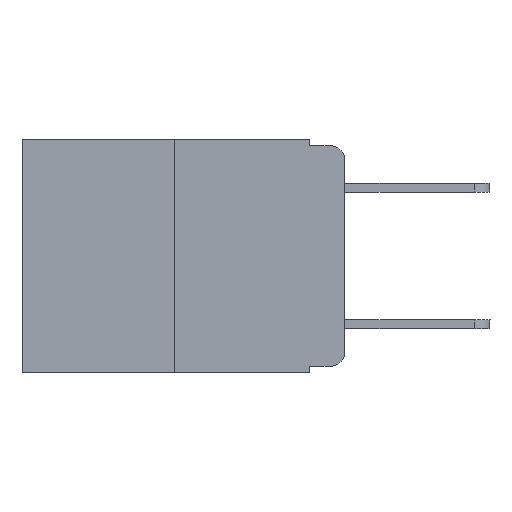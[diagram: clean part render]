
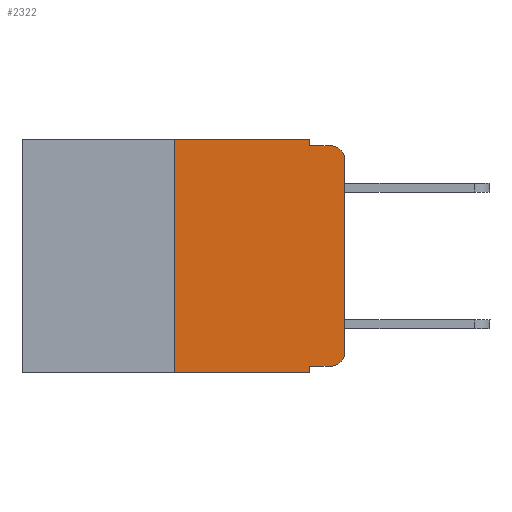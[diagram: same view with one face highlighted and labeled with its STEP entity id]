
A CAD part, left-side view. The second image highlights one B-rep face of the part: STEP entity #2322.
In plain terms, the highlighted planar face has unit normal (-1, 0, 0).
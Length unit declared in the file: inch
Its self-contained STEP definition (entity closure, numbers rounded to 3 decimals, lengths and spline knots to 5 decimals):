
#165 = VERTEX_POINT ( 'NONE', #23968 ) ;
#186 = VERTEX_POINT ( 'NONE', #12737 ) ;
#505 = VECTOR ( 'NONE', #11627, 39.37008 ) ;
#520 = EDGE_CURVE ( 'NONE', #7403, #3630, #7107, .T. ) ;
#828 = DIRECTION ( 'NONE',  ( -1., 0., 0. ) ) ;
#853 = ORIENTED_EDGE ( 'NONE', *, *, #20321, .T. ) ;
#989 = CARTESIAN_POINT ( 'NONE',  ( 0., 0.051, 0. ) ) ;
#1106 = EDGE_CURVE ( 'NONE', #11056, #7403, #2217, .T. ) ;
#1409 = EDGE_CURVE ( 'NONE', #17975, #5112, #13227, .T. ) ;
#1468 = VECTOR ( 'NONE', #15416, 39.37008 ) ;
#1956 = CARTESIAN_POINT ( 'NONE',  ( 0., 0.02, -0.03 ) ) ;
#1979 = VECTOR ( 'NONE', #15609, 39.37008 ) ;
#2217 = LINE ( 'NONE', #9827, #9112 ) ;
#2223 = VECTOR ( 'NONE', #4054, 39.37008 ) ;
#2322 = ADVANCED_FACE ( 'NONE', ( #21819 ), #15921, .F. ) ;
#2340 = CARTESIAN_POINT ( 'NONE',  ( 0., 0.25, -0.343 ) ) ;
#2586 = CARTESIAN_POINT ( 'NONE',  ( 0., 0.051, -0.01 ) ) ;
#2604 = VECTOR ( 'NONE', #2960, 39.37008 ) ;
#2744 = ORIENTED_EDGE ( 'NONE', *, *, #22276, .T. ) ;
#2960 = DIRECTION ( 'NONE',  ( 0., -1., 0. ) ) ;
#3630 = VERTEX_POINT ( 'NONE', #23465 ) ;
#4054 = DIRECTION ( 'NONE',  ( 0., 0., 1. ) ) ;
#4365 = CARTESIAN_POINT ( 'NONE',  ( 0., 0.051, 0. ) ) ;
#4501 = EDGE_CURVE ( 'NONE', #16630, #186, #10085, .T. ) ;
#5112 = VERTEX_POINT ( 'NONE', #14822 ) ;
#5150 = ORIENTED_EDGE ( 'NONE', *, *, #1106, .T. ) ;
#5334 = CARTESIAN_POINT ( 'NONE',  ( 0., 0.051, -0.333 ) ) ;
#5930 = AXIS2_PLACEMENT_3D ( 'NONE', #19654, #17916, #14220 ) ;
#6317 = ORIENTED_EDGE ( 'NONE', *, *, #18060, .F. ) ;
#6747 = ORIENTED_EDGE ( 'NONE', *, *, #4501, .F. ) ;
#6922 = ORIENTED_EDGE ( 'NONE', *, *, #520, .T. ) ;
#7107 = CIRCLE ( 'NONE', #5930, 0.02 ) ;
#7403 = VERTEX_POINT ( 'NONE', #7858 ) ;
#7858 = CARTESIAN_POINT ( 'NONE',  ( 0., 0.02, -0.333 ) ) ;
#8800 = DIRECTION ( 'NONE',  ( 0., 0., 1. ) ) ;
#9112 = VECTOR ( 'NONE', #18946, 39.37008 ) ;
#9827 = CARTESIAN_POINT ( 'NONE',  ( 0., 0.051, -0.333 ) ) ;
#10085 = LINE ( 'NONE', #989, #14245 ) ;
#10498 = DIRECTION ( 'NONE',  ( 0., 0., -1. ) ) ;
#11056 = VERTEX_POINT ( 'NONE', #5334 ) ;
#11627 = DIRECTION ( 'NONE',  ( 0., -1., 0. ) ) ;
#12266 = LINE ( 'NONE', #2586, #1979 ) ;
#12389 = AXIS2_PLACEMENT_3D ( 'NONE', #23678, #14189, #10498 ) ;
#12394 = LINE ( 'NONE', #23743, #2604 ) ;
#12737 = CARTESIAN_POINT ( 'NONE',  ( 0., 0.051, -0.01 ) ) ;
#13227 = LINE ( 'NONE', #13351, #505 ) ;
#13293 = EDGE_CURVE ( 'NONE', #14154, #16630, #12394, .T. ) ;
#13351 = CARTESIAN_POINT ( 'NONE',  ( 0., 0.473, -0.343 ) ) ;
#13363 = LINE ( 'NONE', #16954, #2223 ) ;
#13778 = CARTESIAN_POINT ( 'NONE',  ( 0., 0.02, -0.01 ) ) ;
#14154 = VERTEX_POINT ( 'NONE', #20445 ) ;
#14189 = DIRECTION ( 'NONE',  ( 1., 0., 0. ) ) ;
#14220 = DIRECTION ( 'NONE',  ( 0., 0., -1. ) ) ;
#14245 = VECTOR ( 'NONE', #15750, 39.37008 ) ;
#14822 = CARTESIAN_POINT ( 'NONE',  ( 0., 0.051, -0.343 ) ) ;
#14990 = VERTEX_POINT ( 'NONE', #13778 ) ;
#15416 = DIRECTION ( 'NONE',  ( 0., 0., -1. ) ) ;
#15496 = EDGE_CURVE ( 'NONE', #17975, #14154, #17912, .T. ) ;
#15609 = DIRECTION ( 'NONE',  ( 0., -1., 0. ) ) ;
#15620 = VECTOR ( 'NONE', #8800, 39.37008 ) ;
#15750 = DIRECTION ( 'NONE',  ( 0., 0., -1. ) ) ;
#15921 = PLANE ( 'NONE',  #12389 ) ;
#16630 = VERTEX_POINT ( 'NONE', #22380 ) ;
#16954 = CARTESIAN_POINT ( 'NONE',  ( 0., 0., 0. ) ) ;
#17825 = EDGE_LOOP ( 'NONE', ( #853, #2744, #6317, #6747, #21269, #21698, #18749, #21914, #5150, #6922 ) ) ;
#17912 = LINE ( 'NONE', #22322, #15620 ) ;
#17916 = DIRECTION ( 'NONE',  ( -1., 0., 0. ) ) ;
#17975 = VERTEX_POINT ( 'NONE', #2340 ) ;
#18060 = EDGE_CURVE ( 'NONE', #186, #14990, #12266, .T. ) ;
#18749 = ORIENTED_EDGE ( 'NONE', *, *, #1409, .T. ) ;
#18755 = CIRCLE ( 'NONE', #21113, 0.02 ) ;
#18946 = DIRECTION ( 'NONE',  ( 0., -1., 0. ) ) ;
#19654 = CARTESIAN_POINT ( 'NONE',  ( 0., 0.02, -0.313 ) ) ;
#20321 = EDGE_CURVE ( 'NONE', #3630, #165, #13363, .T. ) ;
#20445 = CARTESIAN_POINT ( 'NONE',  ( 0., 0.25, 0. ) ) ;
#21015 = DIRECTION ( 'NONE',  ( 0., 0., -1. ) ) ;
#21113 = AXIS2_PLACEMENT_3D ( 'NONE', #1956, #828, #21015 ) ;
#21269 = ORIENTED_EDGE ( 'NONE', *, *, #13293, .F. ) ;
#21698 = ORIENTED_EDGE ( 'NONE', *, *, #15496, .F. ) ;
#21819 = FACE_OUTER_BOUND ( 'NONE', #17825, .T. ) ;
#21914 = ORIENTED_EDGE ( 'NONE', *, *, #22607, .F. ) ;
#22276 = EDGE_CURVE ( 'NONE', #165, #14990, #18755, .T. ) ;
#22322 = CARTESIAN_POINT ( 'NONE',  ( 0., 0.25, 0. ) ) ;
#22380 = CARTESIAN_POINT ( 'NONE',  ( 0., 0.051, 0. ) ) ;
#22607 = EDGE_CURVE ( 'NONE', #11056, #5112, #23052, .T. ) ;
#23052 = LINE ( 'NONE', #4365, #1468 ) ;
#23465 = CARTESIAN_POINT ( 'NONE',  ( 0., 0., -0.313 ) ) ;
#23678 = CARTESIAN_POINT ( 'NONE',  ( 0., 0.473, 0. ) ) ;
#23743 = CARTESIAN_POINT ( 'NONE',  ( 0., 0.473, 0. ) ) ;
#23968 = CARTESIAN_POINT ( 'NONE',  ( 0., 0., -0.03 ) ) ;
